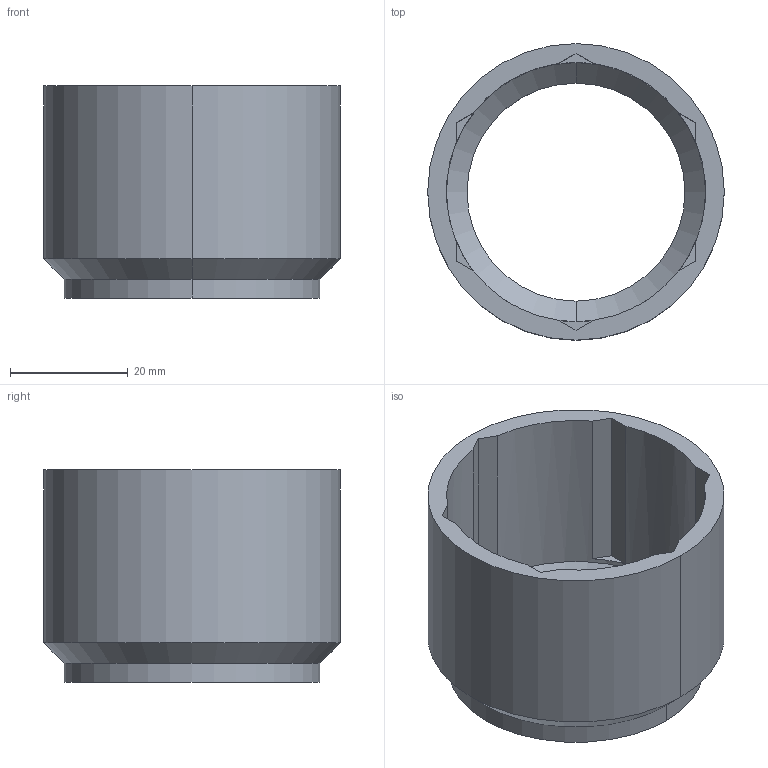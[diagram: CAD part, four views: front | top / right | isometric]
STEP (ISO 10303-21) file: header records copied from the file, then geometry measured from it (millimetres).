
FILE_DESCRIPTION (( 'STEP AP203' ), '1' );
FILE_NAME ('AF-22LR_PP-SB-PRT-001-STEP.STEP', '2020-08-28T10:17:56', ( '' ), ( '' ), 'SwSTEP 2.0', 'SolidWorks 2018', '' );
FILE_SCHEMA (( 'CONFIG_CONTROL_DESIGN' ));
Length unit declared in the file: inch
Products named in the file (1): AF-22LR_PP-SB-PRT-001-STEP
Bounding box: 50.29 x 50.29 x 35.98 mm (x, y, z)
Volume: 15852.9 mm3; surface area: 11855.6 mm2
Topology: 1 solids, 1 shells, 32 faces, 82 edges, 52 vertices
Faces by surface type: plane 20, cylinder 8, cone 4
Entity records: 1053 total; most frequent: DIRECTION 176, CARTESIAN_POINT 167, ORIENTED_EDGE 164, EDGE_CURVE 82, AXIS2_PLACEMENT_3D 61, VECTOR 54, LINE 54, VERTEX_POINT 52
